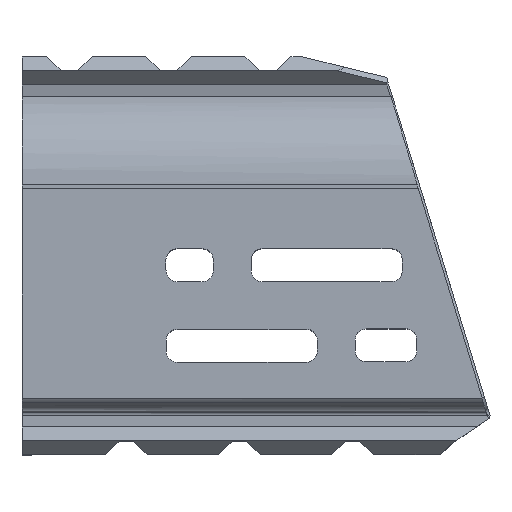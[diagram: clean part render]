
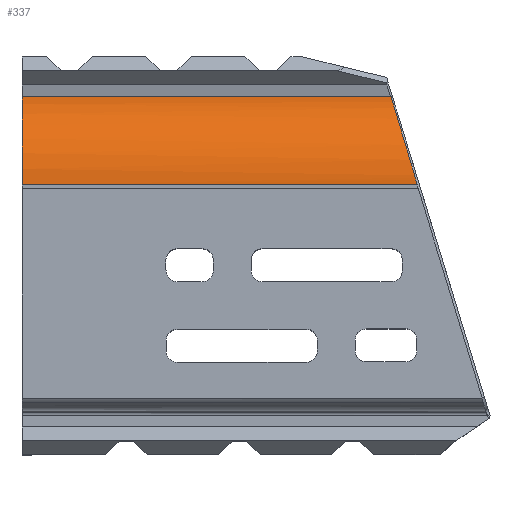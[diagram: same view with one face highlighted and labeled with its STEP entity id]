
A CAD part, top view. The second image highlights one B-rep face of the part: STEP entity #337.
In plain terms, the highlighted cylindrical face has radius 20.1 mm (diameter 40.2 mm), a partial arc.
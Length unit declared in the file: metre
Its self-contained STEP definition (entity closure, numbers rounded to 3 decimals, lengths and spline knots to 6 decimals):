
#337=ADVANCED_FACE('2:47711',(#936),#937,.T.);
#936=FACE_OUTER_BOUND('',#2927,.T.);
#937=CYLINDRICAL_SURFACE('',#2928,0.0201);
#2927=EDGE_LOOP('',(#5413,#5414,#5415,#5416,#5417,#5418));
#2928=AXIS2_PLACEMENT_3D('',#5419,#5420,#5421);
#5413=ORIENTED_EDGE('',*,*,#5762,.F.);
#5414=ORIENTED_EDGE('',*,*,#6265,.F.);
#5415=ORIENTED_EDGE('',*,*,#6257,.F.);
#5416=ORIENTED_EDGE('',*,*,#6256,.T.);
#5417=ORIENTED_EDGE('',*,*,#6253,.F.);
#5418=ORIENTED_EDGE('',*,*,#6250,.F.);
#5419=CARTESIAN_POINT('',(0.011678,0.047361,0.001));
#5420=DIRECTION('',(1.0,-0.0,0.));
#5421=DIRECTION('',(0.,0.0,-1.0));
#5762=EDGE_CURVE('2:47738',#6878,#6880,#6881,.T.);
#6250=EDGE_CURVE('2:47741',#6880,#7617,#7618,.T.);
#6253=EDGE_CURVE('2:50619',#7617,#7620,#7622,.T.);
#6256=EDGE_CURVE('2:58613',#7624,#7620,#7627,.T.);
#6257=EDGE_CURVE('2:54615',#7624,#7628,#7629,.F.);
#6265=EDGE_CURVE('3:13784',#7628,#6878,#7640,.T.);
#6878=VERTEX_POINT('',#8976);
#6880=VERTEX_POINT('',#8979);
#6881=LINE('',#8980,#8981);
#7617=VERTEX_POINT('',#10187);
#7618=CIRCLE('',#10188,0.0201);
#7620=VERTEX_POINT('',#10191);
#7622=LINE('',#10194,#10195);
#7624=VERTEX_POINT('',#10197);
#7627=ELLIPSE('',#10204,0.02876,0.0201);
#7628=VERTEX_POINT('',#10205);
#7629=B_SPLINE_CURVE_WITH_KNOTS('',3,(#10206,#10207,#10208,#10209,#10210,#10211,#10212,#10213,#10214,#10215),.UNSPECIFIED.,.F.,.F.,(4,3,3,4),(-1.570795,-1.246951,-0.505173,-0.379386),.UNSPECIFIED.);
#7640=ELLIPSE('',#10246,0.029724,0.0201);
#8976=CARTESIAN_POINT('',(0.095261,0.047361,0.0211));
#8979=CARTESIAN_POINT('',(0.011678,0.047361,0.0211));
#8980=CARTESIAN_POINT('',(0.053598,0.047361,0.0211));
#8981=VECTOR('',#10795,1.0);
#10187=CARTESIAN_POINT('',(0.011678,0.065991,0.008545));
#10188=AXIS2_PLACEMENT_3D('',#11543,#11544,#11545);
#10191=CARTESIAN_POINT('',(0.08966,0.065991,0.008545));
#10194=CARTESIAN_POINT('',(0.011678,0.065991,0.008545));
#10195=VECTOR('',#11548,1.0);
#10197=CARTESIAN_POINT('',(0.08976,0.066032,0.008444));
#10204=AXIS2_PLACEMENT_3D('',#11550,#11551,#11552);
#10205=CARTESIAN_POINT('',(0.094751,0.049376,0.020999));
#10206=CARTESIAN_POINT('',(0.095355,0.047361,0.0211));
#10207=CARTESIAN_POINT('',(0.094705,0.049531,0.0211));
#10208=CARTESIAN_POINT('',(0.094055,0.051701,0.020746));
#10209=CARTESIAN_POINT('',(0.093438,0.053758,0.020055));
#10210=CARTESIAN_POINT('',(0.092026,0.058469,0.018474));
#10211=CARTESIAN_POINT('',(0.090805,0.062546,0.015077));
#10212=CARTESIAN_POINT('',(0.090084,0.064951,0.010728));
#10213=CARTESIAN_POINT('',(0.089962,0.065359,0.00999));
#10214=CARTESIAN_POINT('',(0.089854,0.06572,0.009227));
#10215=CARTESIAN_POINT('',(0.08976,0.066032,0.008444));
#10246=AXIS2_PLACEMENT_3D('',#11558,#11559,#11560);
#10795=DIRECTION('',(-1.0,0.0,0.));
#11543=CARTESIAN_POINT('',(0.011678,0.047361,0.001));
#11544=DIRECTION('',(-1.0,-0.0,-0.0));
#11545=DIRECTION('',(0.0,0.0,-1.0));
#11548=DIRECTION('',(1.0,-0.0,0.));
#11550=CARTESIAN_POINT('',(0.098799,0.047361,0.001));
#11551=DIRECTION('',(0.699,0.054,0.713));
#11552=DIRECTION('',(0.715,-0.053,-0.697));
#11558=CARTESIAN_POINT('',(0.116279,0.047361,0.001));
#11559=DIRECTION('',(0.676,0.207,0.707));
#11560=DIRECTION('',(0.737,-0.19,-0.649));
